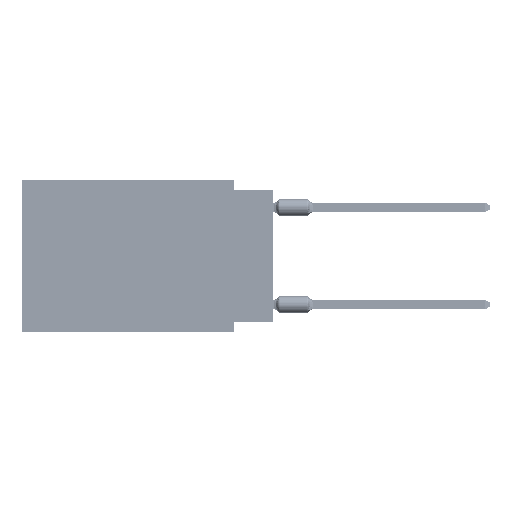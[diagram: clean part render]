
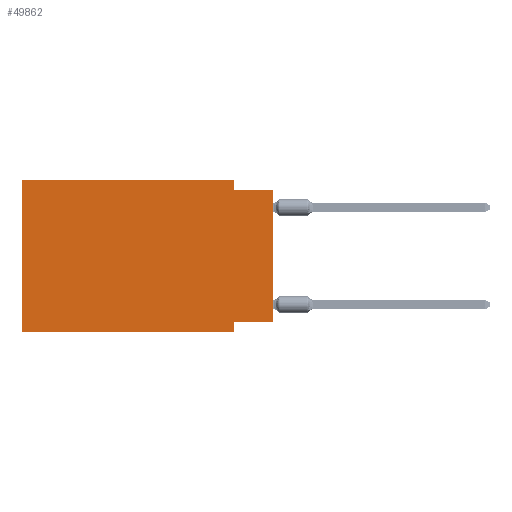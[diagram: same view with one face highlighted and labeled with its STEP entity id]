
A CAD part, left-side view. The second image highlights one B-rep face of the part: STEP entity #49862.
In plain terms, the highlighted planar face has unit normal (-1, 0, 0).
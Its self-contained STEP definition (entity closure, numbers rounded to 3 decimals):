
#418 = DIRECTION ( 'NONE',  ( 0., -1., 0. ) ) ;
#2234 = CARTESIAN_POINT ( 'NONE',  ( 0., 16.383, 0. ) ) ;
#3043 = LINE ( 'NONE', #9285, #55291 ) ;
#3870 = VERTEX_POINT ( 'NONE', #66027 ) ;
#4152 = CARTESIAN_POINT ( 'NONE',  ( 0., 16.383, 0. ) ) ;
#6982 = EDGE_CURVE ( 'NONE', #53695, #53622, #73146, .T. ) ;
#7107 = CARTESIAN_POINT ( 'NONE',  ( 0., 16.383, 0. ) ) ;
#7267 = VERTEX_POINT ( 'NONE', #18176 ) ;
#8846 = CARTESIAN_POINT ( 'NONE',  ( 0., 2.54, 0. ) ) ;
#9285 = CARTESIAN_POINT ( 'NONE',  ( 0., 2.54, -9.906 ) ) ;
#11351 = CARTESIAN_POINT ( 'NONE',  ( 0., 0., -0.635 ) ) ;
#11468 = VERTEX_POINT ( 'NONE', #42507 ) ;
#11592 = DIRECTION ( 'NONE',  ( 0., 0., -1. ) ) ;
#11738 = LINE ( 'NONE', #11351, #31133 ) ;
#13696 = ORIENTED_EDGE ( 'NONE', *, *, #33352, .F. ) ;
#13832 = CARTESIAN_POINT ( 'NONE',  ( 0., 16.383, -9.906 ) ) ;
#16731 = CARTESIAN_POINT ( 'NONE',  ( 0., 0., -9.271 ) ) ;
#17089 = PLANE ( 'NONE',  #74497 ) ;
#18176 = CARTESIAN_POINT ( 'NONE',  ( 0., 0., -0.635 ) ) ;
#20854 = ORIENTED_EDGE ( 'NONE', *, *, #36445, .T. ) ;
#21109 = CARTESIAN_POINT ( 'NONE',  ( 0., 16.383, -9.906 ) ) ;
#21402 = DIRECTION ( 'NONE',  ( 0., 0., -1. ) ) ;
#21831 = CARTESIAN_POINT ( 'NONE',  ( 0., 2.54, -9.906 ) ) ;
#21895 = CARTESIAN_POINT ( 'NONE',  ( 0., 2.54, -0.635 ) ) ;
#22242 = LINE ( 'NONE', #16731, #28274 ) ;
#22522 = ORIENTED_EDGE ( 'NONE', *, *, #70721, .F. ) ;
#23038 = VERTEX_POINT ( 'NONE', #13832 ) ;
#23342 = CARTESIAN_POINT ( 'NONE',  ( 0., 2.54, 0. ) ) ;
#23915 = VERTEX_POINT ( 'NONE', #21831 ) ;
#26095 = DIRECTION ( 'NONE',  ( 0., -1., 0. ) ) ;
#27139 = VERTEX_POINT ( 'NONE', #21895 ) ;
#28274 = VECTOR ( 'NONE', #46524, 1000. ) ;
#29219 = LINE ( 'NONE', #23342, #54177 ) ;
#31133 = VECTOR ( 'NONE', #418, 1000. ) ;
#33296 = VECTOR ( 'NONE', #26095, 1000. ) ;
#33352 = EDGE_CURVE ( 'NONE', #27139, #7267, #11738, .T. ) ;
#33964 = CARTESIAN_POINT ( 'NONE',  ( 0., 16.383, 0. ) ) ;
#35242 = ORIENTED_EDGE ( 'NONE', *, *, #45501, .F. ) ;
#35679 = EDGE_CURVE ( 'NONE', #23038, #53695, #44285, .T. ) ;
#36445 = EDGE_CURVE ( 'NONE', #3870, #7267, #57990, .T. ) ;
#42507 = CARTESIAN_POINT ( 'NONE',  ( 0., 2.54, -9.271 ) ) ;
#44285 = LINE ( 'NONE', #7107, #51253 ) ;
#44640 = DIRECTION ( 'NONE',  ( 0., -1., 0. ) ) ;
#45036 = EDGE_CURVE ( 'NONE', #23038, #23915, #51684, .T. ) ;
#45501 = EDGE_CURVE ( 'NONE', #11468, #23915, #3043, .T. ) ;
#46524 = DIRECTION ( 'NONE',  ( 0., 1., 0. ) ) ;
#46631 = DIRECTION ( 'NONE',  ( 0., 0., 1. ) ) ;
#47019 = CARTESIAN_POINT ( 'NONE',  ( 0., 0., 0. ) ) ;
#49862 = ADVANCED_FACE ( 'NONE', ( #59007 ), #17089, .F. ) ;
#51253 = VECTOR ( 'NONE', #56044, 1000. ) ;
#51684 = LINE ( 'NONE', #21109, #60256 ) ;
#51770 = EDGE_LOOP ( 'NONE', ( #20854, #13696, #22522, #71319, #58019, #74420, #35242, #63654 ) ) ;
#52392 = DIRECTION ( 'NONE',  ( 1., 0., 0. ) ) ;
#53622 = VERTEX_POINT ( 'NONE', #8846 ) ;
#53695 = VERTEX_POINT ( 'NONE', #4152 ) ;
#53768 = VECTOR ( 'NONE', #46631, 1000. ) ;
#54177 = VECTOR ( 'NONE', #11592, 1000. ) ;
#55291 = VECTOR ( 'NONE', #21402, 1000. ) ;
#56044 = DIRECTION ( 'NONE',  ( 0., 0., 1. ) ) ;
#57990 = LINE ( 'NONE', #47019, #53768 ) ;
#58019 = ORIENTED_EDGE ( 'NONE', *, *, #35679, .F. ) ;
#59007 = FACE_OUTER_BOUND ( 'NONE', #51770, .T. ) ;
#60256 = VECTOR ( 'NONE', #44640, 1000. ) ;
#63654 = ORIENTED_EDGE ( 'NONE', *, *, #65552, .F. ) ;
#65552 = EDGE_CURVE ( 'NONE', #3870, #11468, #22242, .T. ) ;
#66027 = CARTESIAN_POINT ( 'NONE',  ( 0., 0., -9.271 ) ) ;
#70721 = EDGE_CURVE ( 'NONE', #53622, #27139, #29219, .T. ) ;
#71319 = ORIENTED_EDGE ( 'NONE', *, *, #6982, .F. ) ;
#73146 = LINE ( 'NONE', #2234, #33296 ) ;
#74420 = ORIENTED_EDGE ( 'NONE', *, *, #45036, .T. ) ;
#74497 = AXIS2_PLACEMENT_3D ( 'NONE', #33964, #52392, #75926 ) ;
#75926 = DIRECTION ( 'NONE',  ( 0., 0., -1. ) ) ;
